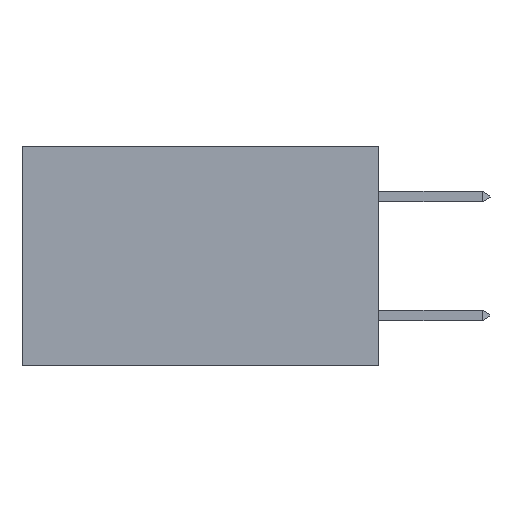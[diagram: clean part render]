
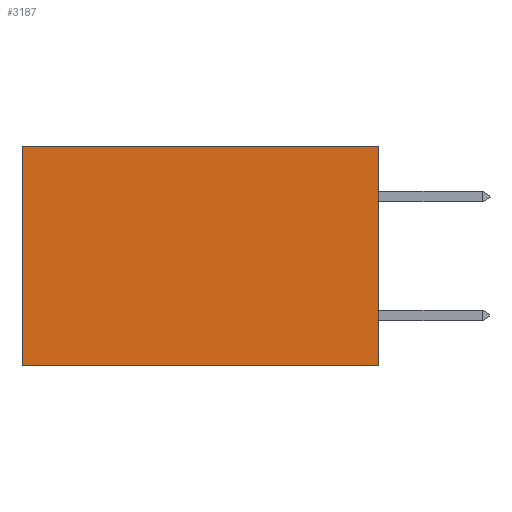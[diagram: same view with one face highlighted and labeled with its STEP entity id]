
A CAD part, left-side view. The second image highlights one B-rep face of the part: STEP entity #3187.
In plain terms, the highlighted planar face has unit normal (-1, 0, 0).
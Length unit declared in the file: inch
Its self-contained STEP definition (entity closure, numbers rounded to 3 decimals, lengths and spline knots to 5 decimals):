
#206 = CARTESIAN_POINT ( 'NONE',  ( 0.298, 0., -0.37 ) ) ;
#548 = VERTEX_POINT ( 'NONE', #206 ) ;
#631 = DIRECTION ( 'NONE',  ( 0., 0., -1. ) ) ;
#1435 = VECTOR ( 'NONE', #10757, 39.37008 ) ;
#1889 = LINE ( 'NONE', #15524, #16182 ) ;
#1972 = CARTESIAN_POINT ( 'NONE',  ( 0.298, 0., 0. ) ) ;
#2040 = LINE ( 'NONE', #2844, #1435 ) ;
#2429 = CARTESIAN_POINT ( 'NONE',  ( 0.298, 0., -0.37 ) ) ;
#2432 = VERTEX_POINT ( 'NONE', #9622 ) ;
#2844 = CARTESIAN_POINT ( 'NONE',  ( 0.298, 0., 0. ) ) ;
#3187 = ADVANCED_FACE ( 'NONE', ( #9067 ), #15054, .F. ) ;
#4050 = EDGE_CURVE ( 'NONE', #548, #6164, #15201, .T. ) ;
#6164 = VERTEX_POINT ( 'NONE', #11332 ) ;
#7173 = DIRECTION ( 'NONE',  ( 1., 0., 0. ) ) ;
#8066 = VECTOR ( 'NONE', #15307, 39.37008 ) ;
#8773 = CARTESIAN_POINT ( 'NONE',  ( 0.298, 0., 0. ) ) ;
#9067 = FACE_OUTER_BOUND ( 'NONE', #10558, .T. ) ;
#9622 = CARTESIAN_POINT ( 'NONE',  ( 0.298, 0., 0. ) ) ;
#9924 = VERTEX_POINT ( 'NONE', #13772 ) ;
#10558 = EDGE_LOOP ( 'NONE', ( #14349, #16408, #11594, #15577 ) ) ;
#10757 = DIRECTION ( 'NONE',  ( 0., 1., 0. ) ) ;
#11238 = DIRECTION ( 'NONE',  ( 0., 0., -1. ) ) ;
#11332 = CARTESIAN_POINT ( 'NONE',  ( 0.298, 0.6, -0.37 ) ) ;
#11594 = ORIENTED_EDGE ( 'NONE', *, *, #15763, .F. ) ;
#11997 = EDGE_CURVE ( 'NONE', #9924, #6164, #1889, .T. ) ;
#13165 = EDGE_CURVE ( 'NONE', #2432, #9924, #2040, .T. ) ;
#13325 = VECTOR ( 'NONE', #11238, 39.37008 ) ;
#13772 = CARTESIAN_POINT ( 'NONE',  ( 0.298, 0.6, 0. ) ) ;
#14181 = DIRECTION ( 'NONE',  ( 0., 0., -1. ) ) ;
#14334 = AXIS2_PLACEMENT_3D ( 'NONE', #1972, #7173, #631 ) ;
#14349 = ORIENTED_EDGE ( 'NONE', *, *, #11997, .T. ) ;
#14963 = LINE ( 'NONE', #8773, #13325 ) ;
#15054 = PLANE ( 'NONE',  #14334 ) ;
#15201 = LINE ( 'NONE', #2429, #8066 ) ;
#15307 = DIRECTION ( 'NONE',  ( 0., 1., 0. ) ) ;
#15524 = CARTESIAN_POINT ( 'NONE',  ( 0.298, 0.6, 0. ) ) ;
#15577 = ORIENTED_EDGE ( 'NONE', *, *, #13165, .T. ) ;
#15763 = EDGE_CURVE ( 'NONE', #2432, #548, #14963, .T. ) ;
#16182 = VECTOR ( 'NONE', #14181, 39.37008 ) ;
#16408 = ORIENTED_EDGE ( 'NONE', *, *, #4050, .F. ) ;
